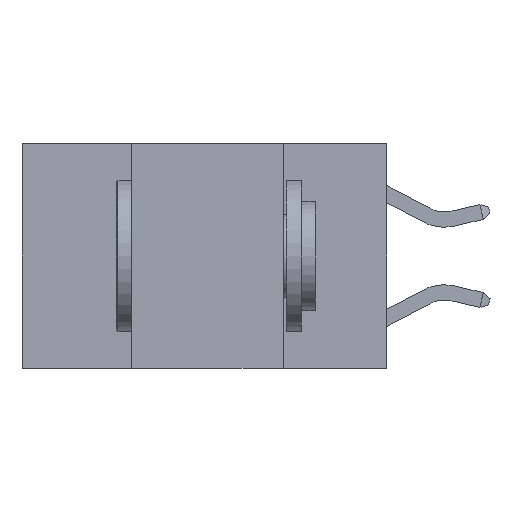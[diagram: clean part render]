
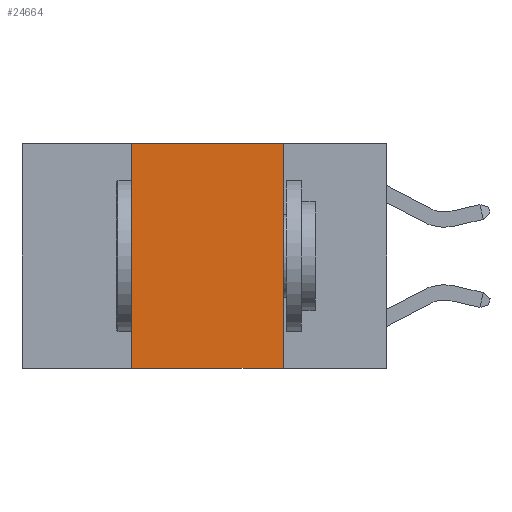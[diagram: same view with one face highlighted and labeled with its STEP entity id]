
A CAD part, left-side view. The second image highlights one B-rep face of the part: STEP entity #24664.
In plain terms, the highlighted planar face has unit normal (-1, 0, 0).
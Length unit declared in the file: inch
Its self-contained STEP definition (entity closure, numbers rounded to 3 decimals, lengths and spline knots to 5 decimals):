
#966 = VECTOR ( 'NONE', #18512, 39.37008 ) ;
#2016 = ORIENTED_EDGE ( 'NONE', *, *, #6318, .F. ) ;
#2163 = CARTESIAN_POINT ( 'NONE',  ( 0., 0.42, -0.37 ) ) ;
#4969 = LINE ( 'NONE', #8250, #26049 ) ;
#5172 = CARTESIAN_POINT ( 'NONE',  ( 0., 0.6, 0. ) ) ;
#5265 = DIRECTION ( 'NONE',  ( 0., 0., -1. ) ) ;
#5600 = ORIENTED_EDGE ( 'NONE', *, *, #10111, .F. ) ;
#5775 = CARTESIAN_POINT ( 'NONE',  ( 0., 0.17, -0.37 ) ) ;
#6318 = EDGE_CURVE ( 'NONE', #18227, #7321, #4969, .T. ) ;
#6548 = CARTESIAN_POINT ( 'NONE',  ( 0., 0.17, 0. ) ) ;
#7321 = VERTEX_POINT ( 'NONE', #21226 ) ;
#8250 = CARTESIAN_POINT ( 'NONE',  ( 0., 0.6, 0. ) ) ;
#8503 = DIRECTION ( 'NONE',  ( 0., 0., -1. ) ) ;
#9632 = DIRECTION ( 'NONE',  ( 0., -1., 0. ) ) ;
#9681 = ORIENTED_EDGE ( 'NONE', *, *, #14213, .F. ) ;
#10111 = EDGE_CURVE ( 'NONE', #18306, #18227, #11820, .T. ) ;
#11451 = VECTOR ( 'NONE', #9632, 39.37008 ) ;
#11820 = LINE ( 'NONE', #24645, #966 ) ;
#13375 = EDGE_CURVE ( 'NONE', #18306, #16236, #21001, .T. ) ;
#13424 = PLANE ( 'NONE',  #21554 ) ;
#14213 = EDGE_CURVE ( 'NONE', #7321, #16236, #16811, .T. ) ;
#16236 = VERTEX_POINT ( 'NONE', #5775 ) ;
#16811 = LINE ( 'NONE', #6548, #21594 ) ;
#16895 = ORIENTED_EDGE ( 'NONE', *, *, #13375, .T. ) ;
#17207 = EDGE_LOOP ( 'NONE', ( #9681, #2016, #5600, #16895 ) ) ;
#17505 = DIRECTION ( 'NONE',  ( 1., 0., 0. ) ) ;
#18030 = FACE_OUTER_BOUND ( 'NONE', #17207, .T. ) ;
#18227 = VERTEX_POINT ( 'NONE', #18237 ) ;
#18237 = CARTESIAN_POINT ( 'NONE',  ( 0., 0.42, 0. ) ) ;
#18306 = VERTEX_POINT ( 'NONE', #2163 ) ;
#18512 = DIRECTION ( 'NONE',  ( 0., 0., 1. ) ) ;
#20461 = DIRECTION ( 'NONE',  ( 0., -1., 0. ) ) ;
#21001 = LINE ( 'NONE', #23899, #11451 ) ;
#21226 = CARTESIAN_POINT ( 'NONE',  ( 0., 0.17, 0. ) ) ;
#21554 = AXIS2_PLACEMENT_3D ( 'NONE', #5172, #17505, #5265 ) ;
#21594 = VECTOR ( 'NONE', #8503, 39.37008 ) ;
#23899 = CARTESIAN_POINT ( 'NONE',  ( 0., 0.6, -0.37 ) ) ;
#24645 = CARTESIAN_POINT ( 'NONE',  ( 0., 0.42, 0. ) ) ;
#24664 = ADVANCED_FACE ( 'NONE', ( #18030 ), #13424, .F. ) ;
#26049 = VECTOR ( 'NONE', #20461, 39.37008 ) ;
